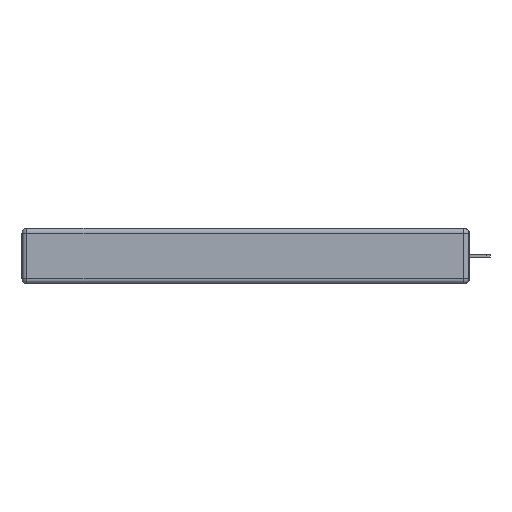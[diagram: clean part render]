
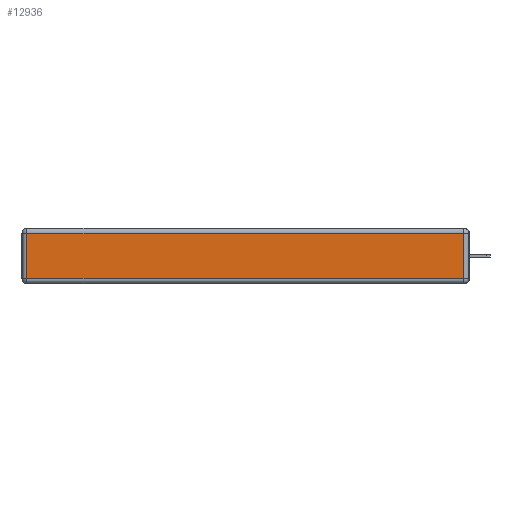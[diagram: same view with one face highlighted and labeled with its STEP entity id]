
A CAD part, left-side view. The second image highlights one B-rep face of the part: STEP entity #12936.
In plain terms, the highlighted planar face has unit normal (-1, 0, 0).
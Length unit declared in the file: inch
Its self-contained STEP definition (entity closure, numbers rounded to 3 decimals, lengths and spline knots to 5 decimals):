
#355 = ORIENTED_EDGE ( 'NONE', *, *, #12864, .T. ) ;
#1730 = CARTESIAN_POINT ( 'NONE',  ( 0., 0.03, -0.313 ) ) ;
#2137 = CARTESIAN_POINT ( 'NONE',  ( 0., 0.03, -0.03 ) ) ;
#2938 = CARTESIAN_POINT ( 'NONE',  ( 0., 2.72, -0.343 ) ) ;
#2976 = VECTOR ( 'NONE', #8429, 39.37008 ) ;
#3756 = CARTESIAN_POINT ( 'NONE',  ( 0., 0., -0.313 ) ) ;
#3931 = DIRECTION ( 'NONE',  ( 0., -1., 0. ) ) ;
#4265 = FACE_OUTER_BOUND ( 'NONE', #11568, .T. ) ;
#4339 = ORIENTED_EDGE ( 'NONE', *, *, #5427, .T. ) ;
#4385 = DIRECTION ( 'NONE',  ( -1., 0., 0. ) ) ;
#5327 = VECTOR ( 'NONE', #3931, 39.37008 ) ;
#5427 = EDGE_CURVE ( 'NONE', #20595, #10639, #6633, .T. ) ;
#6633 = LINE ( 'NONE', #15952, #25919 ) ;
#7496 = LINE ( 'NONE', #20465, #2976 ) ;
#8429 = DIRECTION ( 'NONE',  ( 0., 1., 0. ) ) ;
#8518 = PLANE ( 'NONE',  #22367 ) ;
#8610 = DIRECTION ( 'NONE',  ( 0., 0., 1. ) ) ;
#10639 = VERTEX_POINT ( 'NONE', #2137 ) ;
#10867 = VERTEX_POINT ( 'NONE', #23640 ) ;
#11568 = EDGE_LOOP ( 'NONE', ( #25337, #4339, #355, #12791 ) ) ;
#12791 = ORIENTED_EDGE ( 'NONE', *, *, #25905, .T. ) ;
#12864 = EDGE_CURVE ( 'NONE', #10639, #26519, #7496, .T. ) ;
#12936 = ADVANCED_FACE ( 'NONE', ( #4265 ), #8518, .T. ) ;
#15952 = CARTESIAN_POINT ( 'NONE',  ( 0., 0.03, -0.343 ) ) ;
#16312 = CARTESIAN_POINT ( 'NONE',  ( 0., 2.72, -0.03 ) ) ;
#17265 = VECTOR ( 'NONE', #21323, 39.37008 ) ;
#19873 = LINE ( 'NONE', #2938, #17265 ) ;
#20465 = CARTESIAN_POINT ( 'NONE',  ( 0., 2.75, -0.03 ) ) ;
#20595 = VERTEX_POINT ( 'NONE', #1730 ) ;
#21161 = CARTESIAN_POINT ( 'NONE',  ( 0., 0., -0.343 ) ) ;
#21323 = DIRECTION ( 'NONE',  ( 0., 0., -1. ) ) ;
#21365 = LINE ( 'NONE', #3756, #5327 ) ;
#21973 = EDGE_CURVE ( 'NONE', #10867, #20595, #21365, .T. ) ;
#22367 = AXIS2_PLACEMENT_3D ( 'NONE', #21161, #4385, #8610 ) ;
#23640 = CARTESIAN_POINT ( 'NONE',  ( 0., 2.72, -0.313 ) ) ;
#25337 = ORIENTED_EDGE ( 'NONE', *, *, #21973, .T. ) ;
#25905 = EDGE_CURVE ( 'NONE', #26519, #10867, #19873, .T. ) ;
#25919 = VECTOR ( 'NONE', #26158, 39.37008 ) ;
#26158 = DIRECTION ( 'NONE',  ( 0., 0., 1. ) ) ;
#26519 = VERTEX_POINT ( 'NONE', #16312 ) ;
